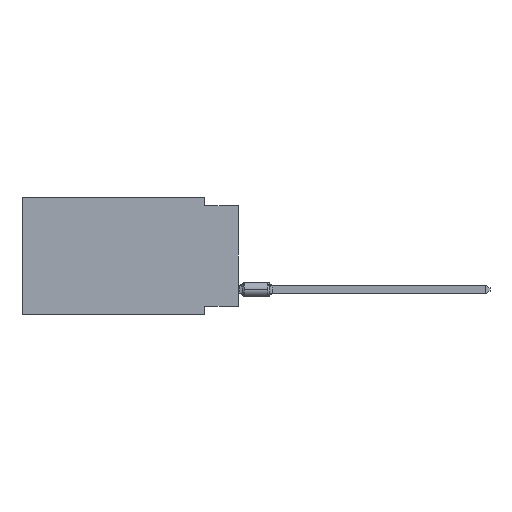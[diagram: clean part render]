
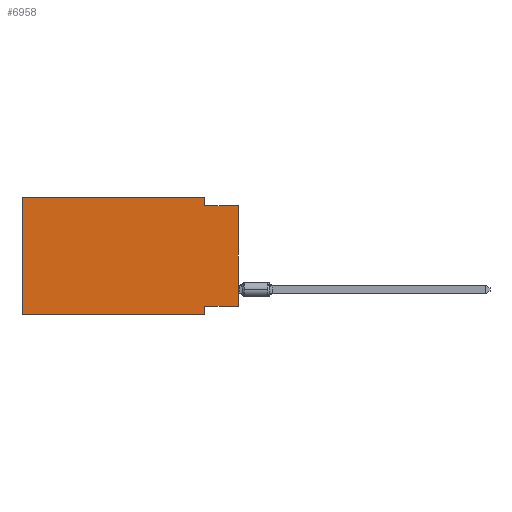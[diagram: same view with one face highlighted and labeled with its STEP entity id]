
A CAD part, left-side view. The second image highlights one B-rep face of the part: STEP entity #6958.
In plain terms, the highlighted planar face has unit normal (-1, 0, 0).
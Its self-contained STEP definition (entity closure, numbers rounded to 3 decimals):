
#207 = EDGE_CURVE ( 'NONE', #2726, #11002, #10988, .T. ) ;
#432 = VECTOR ( 'NONE', #13541, 1000. ) ;
#1188 = VERTEX_POINT ( 'NONE', #18960 ) ;
#1217 = VECTOR ( 'NONE', #8336, 1000. ) ;
#1397 = DIRECTION ( 'NONE',  ( 0., 0., -1. ) ) ;
#1636 = DIRECTION ( 'NONE',  ( 0., -1., 0. ) ) ;
#1648 = VERTEX_POINT ( 'NONE', #7514 ) ;
#1727 = LINE ( 'NONE', #6022, #14586 ) ;
#1785 = VECTOR ( 'NONE', #18990, 1000. ) ;
#2045 = CARTESIAN_POINT ( 'NONE',  ( 0., 2.54, 0. ) ) ;
#2278 = CARTESIAN_POINT ( 'NONE',  ( 0., 0., -8.255 ) ) ;
#2726 = VERTEX_POINT ( 'NONE', #19040 ) ;
#3024 = FACE_OUTER_BOUND ( 'NONE', #6418, .T. ) ;
#3514 = EDGE_CURVE ( 'NONE', #12929, #11509, #12026, .T. ) ;
#3535 = EDGE_CURVE ( 'NONE', #1648, #5741, #8851, .T. ) ;
#3731 = VECTOR ( 'NONE', #16489, 1000. ) ;
#3740 = ORIENTED_EDGE ( 'NONE', *, *, #5334, .T. ) ;
#4086 = CARTESIAN_POINT ( 'NONE',  ( 0., 16.383, 0. ) ) ;
#4161 = EDGE_CURVE ( 'NONE', #11509, #2726, #16102, .T. ) ;
#4813 = ORIENTED_EDGE ( 'NONE', *, *, #207, .F. ) ;
#4836 = ORIENTED_EDGE ( 'NONE', *, *, #5792, .F. ) ;
#5279 = VECTOR ( 'NONE', #12582, 1000. ) ;
#5334 = EDGE_CURVE ( 'NONE', #10372, #1188, #19190, .T. ) ;
#5741 = VERTEX_POINT ( 'NONE', #13003 ) ;
#5792 = EDGE_CURVE ( 'NONE', #10372, #1648, #15988, .T. ) ;
#6022 = CARTESIAN_POINT ( 'NONE',  ( 0., 0., -0.635 ) ) ;
#6331 = ORIENTED_EDGE ( 'NONE', *, *, #8209, .F. ) ;
#6418 = EDGE_LOOP ( 'NONE', ( #3740, #6331, #4813, #19643, #8836, #8417, #6966, #4836 ) ) ;
#6958 = ADVANCED_FACE ( 'NONE', ( #3024 ), #7879, .F. ) ;
#6966 = ORIENTED_EDGE ( 'NONE', *, *, #3535, .F. ) ;
#6968 = CARTESIAN_POINT ( 'NONE',  ( 0., 0., 0. ) ) ;
#7514 = CARTESIAN_POINT ( 'NONE',  ( 0., 2.54, -8.255 ) ) ;
#7879 = PLANE ( 'NONE',  #13380 ) ;
#8209 = EDGE_CURVE ( 'NONE', #11002, #1188, #1727, .T. ) ;
#8336 = DIRECTION ( 'NONE',  ( 0., 1., 0. ) ) ;
#8417 = ORIENTED_EDGE ( 'NONE', *, *, #12601, .T. ) ;
#8836 = ORIENTED_EDGE ( 'NONE', *, *, #3514, .F. ) ;
#8851 = LINE ( 'NONE', #18092, #19286 ) ;
#8972 = LINE ( 'NONE', #10451, #432 ) ;
#9085 = DIRECTION ( 'NONE',  ( 1., 0., 0. ) ) ;
#10372 = VERTEX_POINT ( 'NONE', #15999 ) ;
#10451 = CARTESIAN_POINT ( 'NONE',  ( 0., 16.383, -8.89 ) ) ;
#10723 = VECTOR ( 'NONE', #13225, 1000. ) ;
#10988 = LINE ( 'NONE', #2045, #5279 ) ;
#11002 = VERTEX_POINT ( 'NONE', #12748 ) ;
#11509 = VERTEX_POINT ( 'NONE', #13635 ) ;
#12020 = CARTESIAN_POINT ( 'NONE',  ( 0., 16.383, -8.89 ) ) ;
#12026 = LINE ( 'NONE', #13809, #3731 ) ;
#12454 = CARTESIAN_POINT ( 'NONE',  ( 0., 16.383, 0. ) ) ;
#12582 = DIRECTION ( 'NONE',  ( 0., 0., -1. ) ) ;
#12601 = EDGE_CURVE ( 'NONE', #12929, #5741, #8972, .T. ) ;
#12748 = CARTESIAN_POINT ( 'NONE',  ( 0., 2.54, -0.635 ) ) ;
#12929 = VERTEX_POINT ( 'NONE', #12020 ) ;
#13003 = CARTESIAN_POINT ( 'NONE',  ( 0., 2.54, -8.89 ) ) ;
#13225 = DIRECTION ( 'NONE',  ( 0., 0., 1. ) ) ;
#13380 = AXIS2_PLACEMENT_3D ( 'NONE', #12454, #9085, #15147 ) ;
#13541 = DIRECTION ( 'NONE',  ( 0., -1., 0. ) ) ;
#13635 = CARTESIAN_POINT ( 'NONE',  ( 0., 16.383, 0. ) ) ;
#13809 = CARTESIAN_POINT ( 'NONE',  ( 0., 16.383, 0. ) ) ;
#14586 = VECTOR ( 'NONE', #1636, 1000. ) ;
#15147 = DIRECTION ( 'NONE',  ( 0., 0., -1. ) ) ;
#15988 = LINE ( 'NONE', #2278, #1217 ) ;
#15999 = CARTESIAN_POINT ( 'NONE',  ( 0., 0., -8.255 ) ) ;
#16102 = LINE ( 'NONE', #4086, #1785 ) ;
#16489 = DIRECTION ( 'NONE',  ( 0., 0., 1. ) ) ;
#18092 = CARTESIAN_POINT ( 'NONE',  ( 0., 2.54, -8.89 ) ) ;
#18960 = CARTESIAN_POINT ( 'NONE',  ( 0., 0., -0.635 ) ) ;
#18990 = DIRECTION ( 'NONE',  ( 0., -1., 0. ) ) ;
#19040 = CARTESIAN_POINT ( 'NONE',  ( 0., 2.54, 0. ) ) ;
#19190 = LINE ( 'NONE', #6968, #10723 ) ;
#19286 = VECTOR ( 'NONE', #1397, 1000. ) ;
#19643 = ORIENTED_EDGE ( 'NONE', *, *, #4161, .F. ) ;
